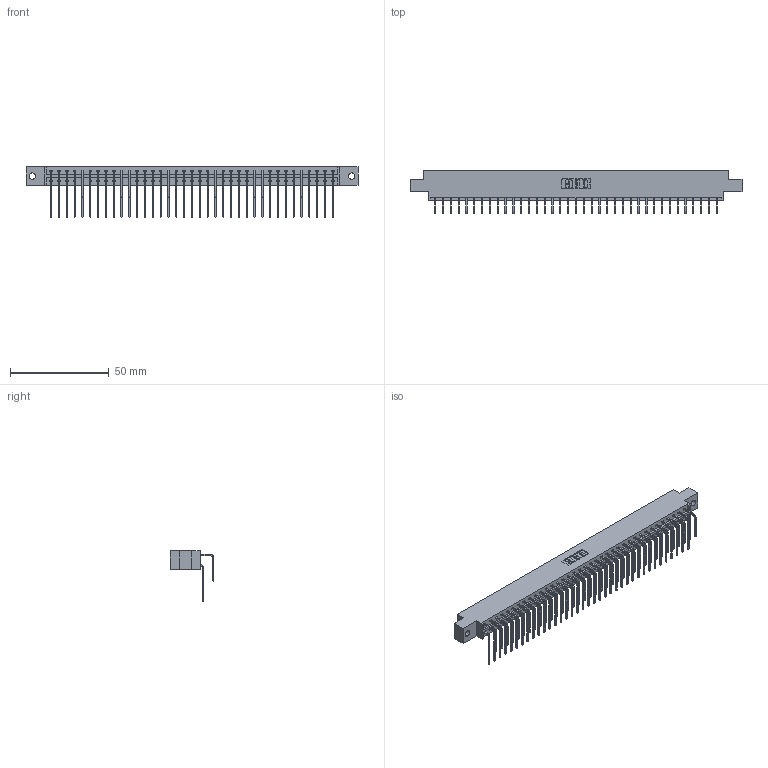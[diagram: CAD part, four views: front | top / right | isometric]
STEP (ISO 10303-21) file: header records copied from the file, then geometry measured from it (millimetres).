
FILE_DESCRIPTION (( 'STEP AP203' ), '1' );
FILE_NAME ('833-074-558-802.STEP', '2020-06-05T17:23:22', ( '' ), ( '' ), 'SwSTEP 2.0', 'SolidWorks 2020', '' );
FILE_SCHEMA (( 'CONFIG_CONTROL_DESIGN' ));
Length unit declared in the file: inch
Products named in the file (4): 345-292-001_558 559 Tail - 1; 833-074-558-802; 833 Part_Offset - .128 Dia; 345-292-001_558 Tail - 2
Assembly tree (75 placements, depth 2):
  833-074-558-802
    833 Part_Offset - .128 Dia
    345-292-001_558 559 Tail - 1  x37
    345-292-001_558 Tail - 2  x37
Bounding box: 168.15 x 22.17 x 25.53 mm (x, y, z)
Volume: 17282.6 mm3; surface area: 22452.4 mm2
Topology: 75 solids, 75 shells, 4114 faces, 12237 edges, 8058 vertices
Faces by surface type: plane 2886, cylinder 1228
Entity records: 26369 total; most frequent: CARTESIAN_POINT 4429, ORIENTED_EDGE 4314, DIRECTION 3773, EDGE_CURVE 2157, VECTOR 1989, LINE 1989, VERTEX_POINT 1434, AXIS2_PLACEMENT_3D 892
